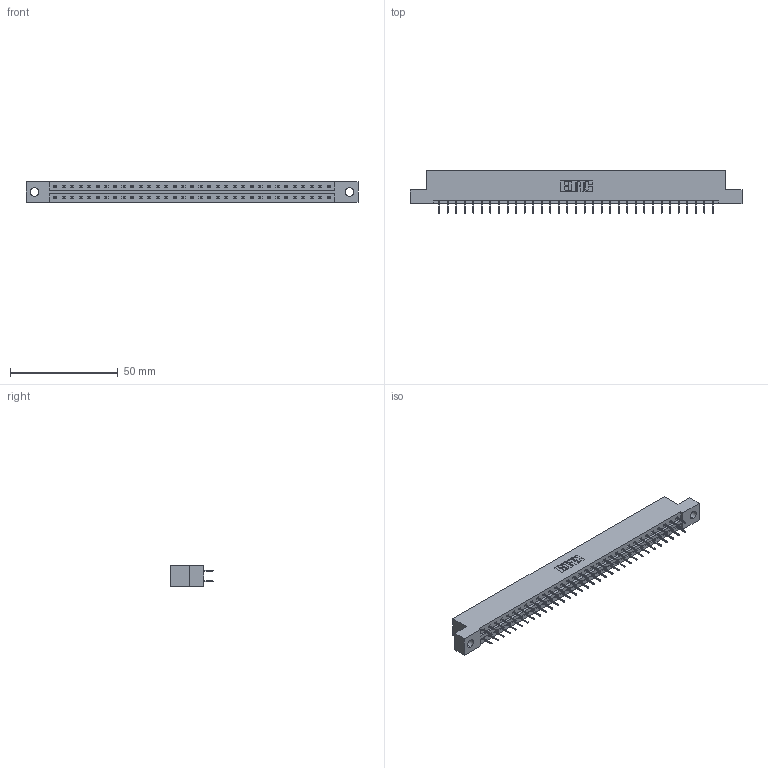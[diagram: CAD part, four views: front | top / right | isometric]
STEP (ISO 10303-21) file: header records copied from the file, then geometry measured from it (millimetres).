
FILE_DESCRIPTION (( 'STEP AP203' ), '1' );
FILE_NAME ('387-066-524-204.STEP', '2018-09-21T09:34:42', ( '' ), ( '' ), 'SwSTEP 2.0', 'SolidWorks 2016', '' );
FILE_SCHEMA (( 'CONFIG_CONTROL_DESIGN' ));
Length unit declared in the file: inch
Products named in the file (3): 337 Part_Flush Mounting Lugs - 0.156 Dia-TH; 345-292-001_345-293-124; 387-066-524-204
Assembly tree (67 placements, depth 2):
  387-066-524-204
    337 Part_Flush Mounting Lugs - 0.156 Dia-TH
    345-292-001_345-293-124  x66
Bounding box: 153.77 x 19.69 x 9.4 mm (x, y, z)
Volume: 15898.1 mm3; surface area: 17373.5 mm2
Topology: 67 solids, 67 shells, 3942 faces, 11201 edges, 7202 vertices
Faces by surface type: plane 2974, cylinder 968
Entity records: 26827 total; most frequent: CARTESIAN_POINT 4526, ORIENTED_EDGE 4462, DIRECTION 3867, EDGE_CURVE 2231, LINE 2107, VECTOR 2107, VERTEX_POINT 1482, AXIS2_PLACEMENT_3D 880
